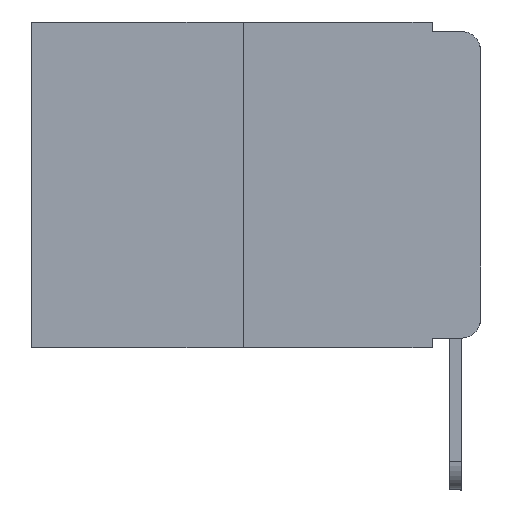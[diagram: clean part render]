
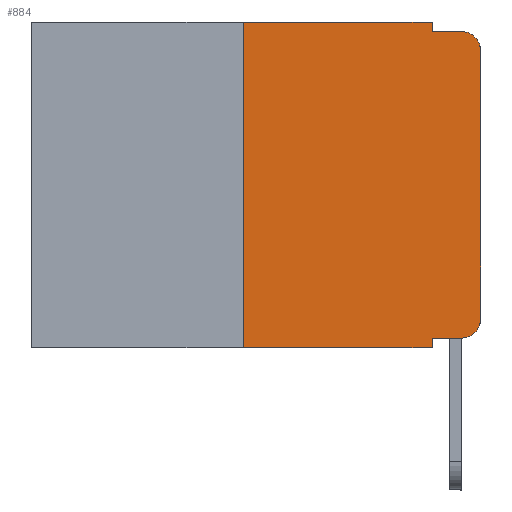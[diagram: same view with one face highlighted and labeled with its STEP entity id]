
A CAD part, left-side view. The second image highlights one B-rep face of the part: STEP entity #884.
In plain terms, the highlighted planar face has unit normal (-1, 0, 0).
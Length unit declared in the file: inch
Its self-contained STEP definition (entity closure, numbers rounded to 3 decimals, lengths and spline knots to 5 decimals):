
#29 = LINE ( 'NONE', #8426, #5473 ) ;
#481 = FACE_OUTER_BOUND ( 'NONE', #24849, .T. ) ;
#884 = ADVANCED_FACE ( 'NONE', ( #481 ), #1027, .F. ) ;
#1027 = PLANE ( 'NONE',  #18613 ) ;
#1561 = DIRECTION ( 'NONE',  ( 0., 0., -1. ) ) ;
#1695 = CARTESIAN_POINT ( 'NONE',  ( 0., 0.051, 0. ) ) ;
#1830 = EDGE_CURVE ( 'NONE', #12736, #17058, #14987, .T. ) ;
#2190 = LINE ( 'NONE', #13154, #21434 ) ;
#2717 = DIRECTION ( 'NONE',  ( 0., -1., 0. ) ) ;
#2790 = LINE ( 'NONE', #9238, #7115 ) ;
#3042 = VERTEX_POINT ( 'NONE', #19638 ) ;
#3349 = EDGE_CURVE ( 'NONE', #12491, #12213, #18678, .T. ) ;
#3781 = ORIENTED_EDGE ( 'NONE', *, *, #7205, .F. ) ;
#4101 = DIRECTION ( 'NONE',  ( 0., 0., 1. ) ) ;
#4149 = CARTESIAN_POINT ( 'NONE',  ( 0., 0.25, 0. ) ) ;
#4359 = DIRECTION ( 'NONE',  ( -1., 0., 0. ) ) ;
#4421 = LINE ( 'NONE', #4149, #15787 ) ;
#4425 = DIRECTION ( 'NONE',  ( 0., -1., 0. ) ) ;
#4643 = EDGE_CURVE ( 'NONE', #24449, #22999, #2790, .T. ) ;
#4897 = CARTESIAN_POINT ( 'NONE',  ( 0., 0., -0.313 ) ) ;
#5022 = VERTEX_POINT ( 'NONE', #19674 ) ;
#5129 = DIRECTION ( 'NONE',  ( 1., 0., 0. ) ) ;
#5146 = AXIS2_PLACEMENT_3D ( 'NONE', #21102, #19171, #8733 ) ;
#5473 = VECTOR ( 'NONE', #4425, 39.37008 ) ;
#7115 = VECTOR ( 'NONE', #17765, 39.37008 ) ;
#7205 = EDGE_CURVE ( 'NONE', #10835, #19705, #9573, .T. ) ;
#8162 = AXIS2_PLACEMENT_3D ( 'NONE', #8356, #4359, #10274 ) ;
#8191 = CARTESIAN_POINT ( 'NONE',  ( 0., 0.051, -0.333 ) ) ;
#8356 = CARTESIAN_POINT ( 'NONE',  ( 0., 0.02, -0.03 ) ) ;
#8426 = CARTESIAN_POINT ( 'NONE',  ( 0., 0.051, -0.333 ) ) ;
#8465 = CARTESIAN_POINT ( 'NONE',  ( 0., 0.051, -0.01 ) ) ;
#8486 = VECTOR ( 'NONE', #24271, 39.37008 ) ;
#8733 = DIRECTION ( 'NONE',  ( 0., 0., -1. ) ) ;
#8967 = EDGE_CURVE ( 'NONE', #12736, #5022, #29, .T. ) ;
#9059 = CARTESIAN_POINT ( 'NONE',  ( 0., 0.051, 0. ) ) ;
#9238 = CARTESIAN_POINT ( 'NONE',  ( 0., 0.051, -0.01 ) ) ;
#9573 = LINE ( 'NONE', #24546, #8486 ) ;
#9880 = EDGE_CURVE ( 'NONE', #12213, #22999, #12533, .T. ) ;
#10274 = DIRECTION ( 'NONE',  ( 0., 0., -1. ) ) ;
#10835 = VERTEX_POINT ( 'NONE', #25815 ) ;
#11216 = ORIENTED_EDGE ( 'NONE', *, *, #8967, .T. ) ;
#11566 = ORIENTED_EDGE ( 'NONE', *, *, #12807, .T. ) ;
#11720 = LINE ( 'NONE', #1695, #15843 ) ;
#11885 = ORIENTED_EDGE ( 'NONE', *, *, #13848, .T. ) ;
#12213 = VERTEX_POINT ( 'NONE', #22263 ) ;
#12349 = CARTESIAN_POINT ( 'NONE',  ( 0., 0., 0. ) ) ;
#12491 = VERTEX_POINT ( 'NONE', #4897 ) ;
#12529 = DIRECTION ( 'NONE',  ( 0., 0., 1. ) ) ;
#12533 = CIRCLE ( 'NONE', #8162, 0.02 ) ;
#12736 = VERTEX_POINT ( 'NONE', #8191 ) ;
#12807 = EDGE_CURVE ( 'NONE', #5022, #12491, #18335, .T. ) ;
#13006 = ORIENTED_EDGE ( 'NONE', *, *, #3349, .T. ) ;
#13110 = DIRECTION ( 'NONE',  ( 0., 0., -1. ) ) ;
#13154 = CARTESIAN_POINT ( 'NONE',  ( 0., 0.473, -0.343 ) ) ;
#13848 = EDGE_CURVE ( 'NONE', #3042, #17058, #2190, .T. ) ;
#14508 = ORIENTED_EDGE ( 'NONE', *, *, #4643, .F. ) ;
#14987 = LINE ( 'NONE', #9059, #20846 ) ;
#15787 = VECTOR ( 'NONE', #12529, 39.37008 ) ;
#15843 = VECTOR ( 'NONE', #1561, 39.37008 ) ;
#16531 = VECTOR ( 'NONE', #4101, 39.37008 ) ;
#17058 = VERTEX_POINT ( 'NONE', #19341 ) ;
#17761 = ORIENTED_EDGE ( 'NONE', *, *, #1830, .F. ) ;
#17765 = DIRECTION ( 'NONE',  ( 0., -1., 0. ) ) ;
#18335 = CIRCLE ( 'NONE', #5146, 0.02 ) ;
#18613 = AXIS2_PLACEMENT_3D ( 'NONE', #21899, #5129, #13110 ) ;
#18678 = LINE ( 'NONE', #12349, #16531 ) ;
#19171 = DIRECTION ( 'NONE',  ( -1., 0., 0. ) ) ;
#19341 = CARTESIAN_POINT ( 'NONE',  ( 0., 0.051, -0.343 ) ) ;
#19638 = CARTESIAN_POINT ( 'NONE',  ( 0., 0.25, -0.343 ) ) ;
#19674 = CARTESIAN_POINT ( 'NONE',  ( 0., 0.02, -0.333 ) ) ;
#19705 = VERTEX_POINT ( 'NONE', #24003 ) ;
#20813 = EDGE_CURVE ( 'NONE', #3042, #10835, #4421, .T. ) ;
#20846 = VECTOR ( 'NONE', #21297, 39.37008 ) ;
#21102 = CARTESIAN_POINT ( 'NONE',  ( 0., 0.02, -0.313 ) ) ;
#21297 = DIRECTION ( 'NONE',  ( 0., 0., -1. ) ) ;
#21434 = VECTOR ( 'NONE', #2717, 39.37008 ) ;
#21899 = CARTESIAN_POINT ( 'NONE',  ( 0., 0.473, 0. ) ) ;
#22263 = CARTESIAN_POINT ( 'NONE',  ( 0., 0., -0.03 ) ) ;
#22541 = ORIENTED_EDGE ( 'NONE', *, *, #9880, .T. ) ;
#22999 = VERTEX_POINT ( 'NONE', #25910 ) ;
#23094 = ORIENTED_EDGE ( 'NONE', *, *, #23473, .F. ) ;
#23473 = EDGE_CURVE ( 'NONE', #19705, #24449, #11720, .T. ) ;
#24003 = CARTESIAN_POINT ( 'NONE',  ( 0., 0.051, 0. ) ) ;
#24271 = DIRECTION ( 'NONE',  ( 0., -1., 0. ) ) ;
#24449 = VERTEX_POINT ( 'NONE', #8465 ) ;
#24546 = CARTESIAN_POINT ( 'NONE',  ( 0., 0.473, 0. ) ) ;
#24797 = ORIENTED_EDGE ( 'NONE', *, *, #20813, .F. ) ;
#24849 = EDGE_LOOP ( 'NONE', ( #13006, #22541, #14508, #23094, #3781, #24797, #11885, #17761, #11216, #11566 ) ) ;
#25815 = CARTESIAN_POINT ( 'NONE',  ( 0., 0.25, 0. ) ) ;
#25910 = CARTESIAN_POINT ( 'NONE',  ( 0., 0.02, -0.01 ) ) ;
